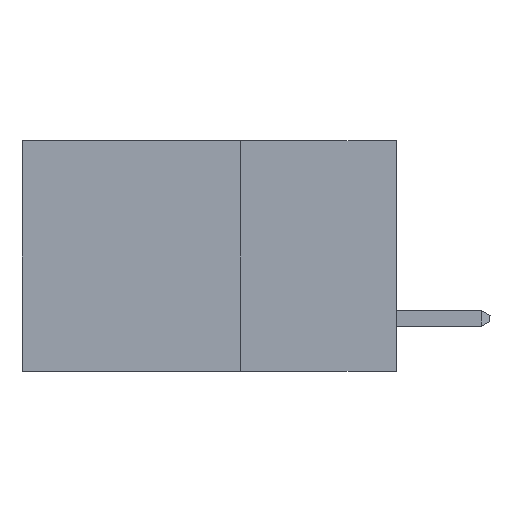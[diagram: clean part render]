
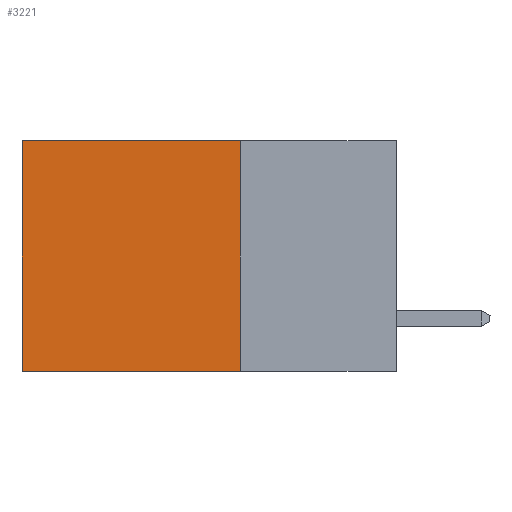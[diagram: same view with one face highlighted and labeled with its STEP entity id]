
A CAD part, left-side view. The second image highlights one B-rep face of the part: STEP entity #3221.
In plain terms, the highlighted planar face has unit normal (-1, 0, 0).
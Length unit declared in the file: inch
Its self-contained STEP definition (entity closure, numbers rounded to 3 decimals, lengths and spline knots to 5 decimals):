
#561 = VECTOR ( 'NONE', #12641, 39.37008 ) ;
#1247 = LINE ( 'NONE', #7097, #6506 ) ;
#1312 = LINE ( 'NONE', #6855, #11172 ) ;
#1414 = ORIENTED_EDGE ( 'NONE', *, *, #11591, .T. ) ;
#1621 = VERTEX_POINT ( 'NONE', #7664 ) ;
#1710 = DIRECTION ( 'NONE',  ( 0., 1., 0. ) ) ;
#1779 = VERTEX_POINT ( 'NONE', #12300 ) ;
#2020 = CARTESIAN_POINT ( 'NONE',  ( 0.2615, 0.25, -0.37 ) ) ;
#2542 = AXIS2_PLACEMENT_3D ( 'NONE', #7801, #4061, #3874 ) ;
#3089 = EDGE_LOOP ( 'NONE', ( #6342, #8844, #4021, #1414 ) ) ;
#3221 = ADVANCED_FACE ( 'NONE', ( #10878 ), #7799, .F. ) ;
#3409 = EDGE_CURVE ( 'NONE', #1779, #12515, #9576, .T. ) ;
#3436 = EDGE_CURVE ( 'NONE', #1621, #11486, #1247, .T. ) ;
#3619 = LINE ( 'NONE', #5328, #561 ) ;
#3874 = DIRECTION ( 'NONE',  ( 0., 0., -1. ) ) ;
#4021 = ORIENTED_EDGE ( 'NONE', *, *, #3436, .F. ) ;
#4061 = DIRECTION ( 'NONE',  ( 1., 0., 0. ) ) ;
#5328 = CARTESIAN_POINT ( 'NONE',  ( 0.2615, 0.25, 0. ) ) ;
#6342 = ORIENTED_EDGE ( 'NONE', *, *, #3409, .T. ) ;
#6360 = CARTESIAN_POINT ( 'NONE',  ( 0.2615, 0.6, -0.37 ) ) ;
#6506 = VECTOR ( 'NONE', #7576, 39.37008 ) ;
#6855 = CARTESIAN_POINT ( 'NONE',  ( 0.2615, 0.25, -0.37 ) ) ;
#7097 = CARTESIAN_POINT ( 'NONE',  ( 0.2615, 0.25, -0.37 ) ) ;
#7110 = VECTOR ( 'NONE', #9776, 39.37008 ) ;
#7576 = DIRECTION ( 'NONE',  ( 0., 0., -1. ) ) ;
#7664 = CARTESIAN_POINT ( 'NONE',  ( 0.2615, 0.25, 0. ) ) ;
#7772 = EDGE_CURVE ( 'NONE', #11486, #12515, #1312, .T. ) ;
#7799 = PLANE ( 'NONE',  #2542 ) ;
#7801 = CARTESIAN_POINT ( 'NONE',  ( 0.2615, 0.25, -0.37 ) ) ;
#8844 = ORIENTED_EDGE ( 'NONE', *, *, #7772, .F. ) ;
#9237 = CARTESIAN_POINT ( 'NONE',  ( 0.2615, 0.6, -0.37 ) ) ;
#9576 = LINE ( 'NONE', #6360, #7110 ) ;
#9776 = DIRECTION ( 'NONE',  ( 0., 0., -1. ) ) ;
#10878 = FACE_OUTER_BOUND ( 'NONE', #3089, .T. ) ;
#11172 = VECTOR ( 'NONE', #1710, 39.37008 ) ;
#11486 = VERTEX_POINT ( 'NONE', #2020 ) ;
#11591 = EDGE_CURVE ( 'NONE', #1621, #1779, #3619, .T. ) ;
#12300 = CARTESIAN_POINT ( 'NONE',  ( 0.2615, 0.6, 0. ) ) ;
#12515 = VERTEX_POINT ( 'NONE', #9237 ) ;
#12641 = DIRECTION ( 'NONE',  ( 0., 1., 0. ) ) ;
